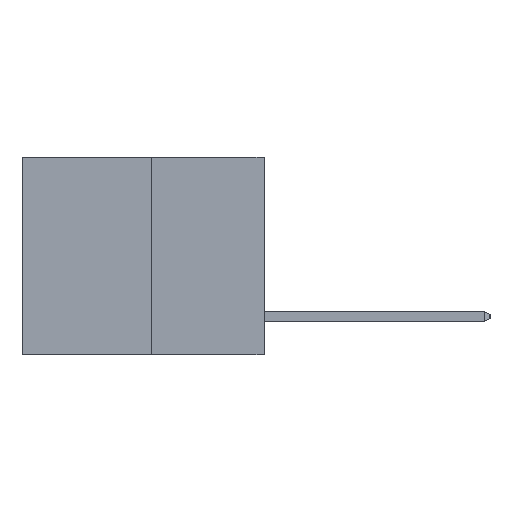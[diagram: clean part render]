
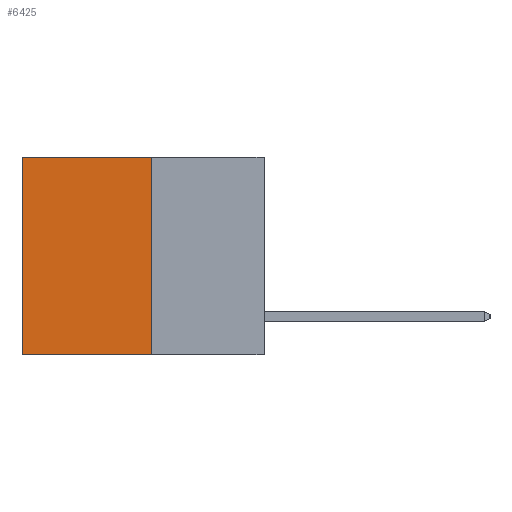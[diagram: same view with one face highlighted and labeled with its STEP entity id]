
A CAD part, left-side view. The second image highlights one B-rep face of the part: STEP entity #6425.
In plain terms, the highlighted planar face has unit normal (-1, 0, 0).
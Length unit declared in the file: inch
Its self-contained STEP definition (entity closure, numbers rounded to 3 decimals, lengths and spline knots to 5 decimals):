
#189 = VECTOR ( 'NONE', #18714, 39.37008 ) ;
#217 = CARTESIAN_POINT ( 'NONE',  ( 0.3165, 0.6, 0. ) ) ;
#516 = EDGE_CURVE ( 'NONE', #7800, #7784, #12651, .T. ) ;
#3620 = CARTESIAN_POINT ( 'NONE',  ( 0.3165, 0.6, -0.49 ) ) ;
#3733 = VECTOR ( 'NONE', #11054, 39.37008 ) ;
#4004 = DIRECTION ( 'NONE',  ( 0., 0., -1. ) ) ;
#4154 = ORIENTED_EDGE ( 'NONE', *, *, #17064, .F. ) ;
#4514 = CARTESIAN_POINT ( 'NONE',  ( 0.3165, 0.28, -0.49 ) ) ;
#4647 = CARTESIAN_POINT ( 'NONE',  ( 0.3165, 0.28, 0. ) ) ;
#4720 = EDGE_CURVE ( 'NONE', #18326, #14396, #10799, .T. ) ;
#4797 = DIRECTION ( 'NONE',  ( 0., 1., 0. ) ) ;
#5799 = ORIENTED_EDGE ( 'NONE', *, *, #516, .F. ) ;
#6425 = ADVANCED_FACE ( 'NONE', ( #15834 ), #8873, .F. ) ;
#6602 = EDGE_LOOP ( 'NONE', ( #10736, #5799, #4154, #11429 ) ) ;
#7784 = VERTEX_POINT ( 'NONE', #3620 ) ;
#7800 = VERTEX_POINT ( 'NONE', #18269 ) ;
#8653 = CARTESIAN_POINT ( 'NONE',  ( 0.3165, 0.28, -0.49 ) ) ;
#8873 = PLANE ( 'NONE',  #16003 ) ;
#10736 = ORIENTED_EDGE ( 'NONE', *, *, #16526, .T. ) ;
#10799 = LINE ( 'NONE', #4647, #15858 ) ;
#11054 = DIRECTION ( 'NONE',  ( 0., 0., -1. ) ) ;
#11429 = ORIENTED_EDGE ( 'NONE', *, *, #4720, .T. ) ;
#12651 = LINE ( 'NONE', #4514, #18444 ) ;
#14013 = CARTESIAN_POINT ( 'NONE',  ( 0.3165, 0.28, 0. ) ) ;
#14396 = VERTEX_POINT ( 'NONE', #217 ) ;
#15798 = DIRECTION ( 'NONE',  ( 0., 1., 0. ) ) ;
#15834 = FACE_OUTER_BOUND ( 'NONE', #6602, .T. ) ;
#15858 = VECTOR ( 'NONE', #4797, 39.37008 ) ;
#15983 = CARTESIAN_POINT ( 'NONE',  ( 0.3165, 0.28, -0.49 ) ) ;
#16003 = AXIS2_PLACEMENT_3D ( 'NONE', #8653, #20077, #4004 ) ;
#16056 = CARTESIAN_POINT ( 'NONE',  ( 0.3165, 0.6, -0.49 ) ) ;
#16526 = EDGE_CURVE ( 'NONE', #14396, #7784, #19115, .T. ) ;
#17064 = EDGE_CURVE ( 'NONE', #18326, #7800, #19344, .T. ) ;
#18269 = CARTESIAN_POINT ( 'NONE',  ( 0.3165, 0.28, -0.49 ) ) ;
#18326 = VERTEX_POINT ( 'NONE', #14013 ) ;
#18444 = VECTOR ( 'NONE', #15798, 39.37008 ) ;
#18714 = DIRECTION ( 'NONE',  ( 0., 0., -1. ) ) ;
#19115 = LINE ( 'NONE', #16056, #3733 ) ;
#19344 = LINE ( 'NONE', #15983, #189 ) ;
#20077 = DIRECTION ( 'NONE',  ( 1., 0., 0. ) ) ;
